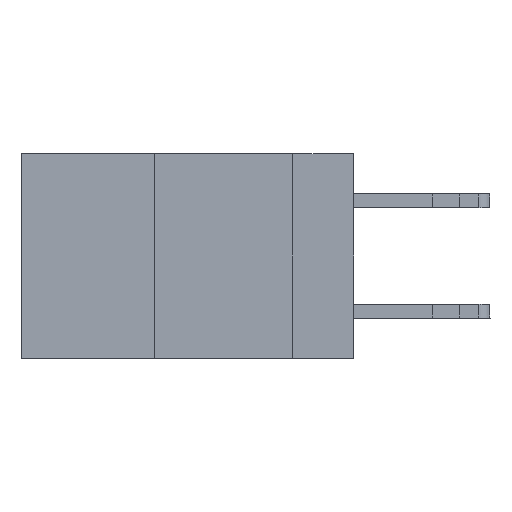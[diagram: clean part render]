
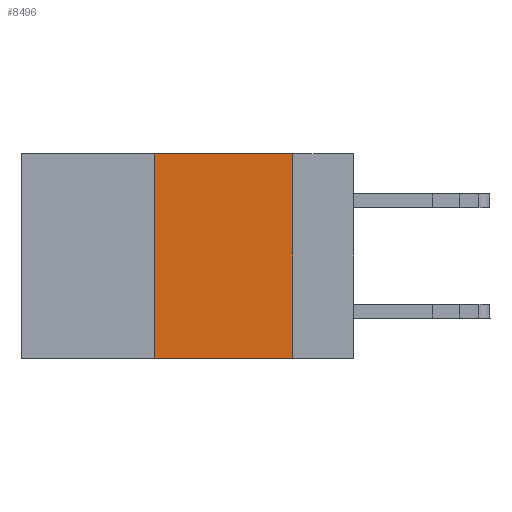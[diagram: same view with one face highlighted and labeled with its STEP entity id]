
A CAD part, left-side view. The second image highlights one B-rep face of the part: STEP entity #8496.
In plain terms, the highlighted planar face has unit normal (-1, 0, 0).
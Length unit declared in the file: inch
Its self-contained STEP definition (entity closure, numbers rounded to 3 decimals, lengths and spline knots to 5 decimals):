
#529 = CARTESIAN_POINT ( 'NONE',  ( 0., 0.36, 0. ) ) ;
#3308 = AXIS2_PLACEMENT_3D ( 'NONE', #15281, #18104, #31017 ) ;
#3557 = VERTEX_POINT ( 'NONE', #18134 ) ;
#4475 = CARTESIAN_POINT ( 'NONE',  ( 0., 0.6, 0. ) ) ;
#4531 = EDGE_LOOP ( 'NONE', ( #20678, #22236, #29000, #11725 ) ) ;
#5773 = VECTOR ( 'NONE', #17639, 39.37008 ) ;
#7805 = VECTOR ( 'NONE', #26830, 39.37008 ) ;
#8262 = LINE ( 'NONE', #529, #11926 ) ;
#8496 = ADVANCED_FACE ( 'NONE', ( #32356 ), #33274, .F. ) ;
#8916 = CARTESIAN_POINT ( 'NONE',  ( 0., 0.11, -0.37 ) ) ;
#10449 = DIRECTION ( 'NONE',  ( 0., 0., 1. ) ) ;
#11725 = ORIENTED_EDGE ( 'NONE', *, *, #25978, .T. ) ;
#11751 = EDGE_CURVE ( 'NONE', #28213, #17127, #28476, .T. ) ;
#11926 = VECTOR ( 'NONE', #10449, 39.37008 ) ;
#12063 = LINE ( 'NONE', #23306, #20612 ) ;
#15281 = CARTESIAN_POINT ( 'NONE',  ( 0., 0.6, 0. ) ) ;
#17127 = VERTEX_POINT ( 'NONE', #23658 ) ;
#17639 = DIRECTION ( 'NONE',  ( 0., -1., 0. ) ) ;
#18104 = DIRECTION ( 'NONE',  ( 1., 0., 0. ) ) ;
#18134 = CARTESIAN_POINT ( 'NONE',  ( 0., 0.36, -0.37 ) ) ;
#20462 = DIRECTION ( 'NONE',  ( 0., 0., -1. ) ) ;
#20612 = VECTOR ( 'NONE', #20462, 39.37008 ) ;
#20678 = ORIENTED_EDGE ( 'NONE', *, *, #23579, .F. ) ;
#22236 = ORIENTED_EDGE ( 'NONE', *, *, #11751, .F. ) ;
#23306 = CARTESIAN_POINT ( 'NONE',  ( 0., 0.11, 0. ) ) ;
#23579 = EDGE_CURVE ( 'NONE', #17127, #25927, #12063, .T. ) ;
#23658 = CARTESIAN_POINT ( 'NONE',  ( 0., 0.11, 0. ) ) ;
#25927 = VERTEX_POINT ( 'NONE', #8916 ) ;
#25978 = EDGE_CURVE ( 'NONE', #3557, #25927, #29318, .T. ) ;
#26830 = DIRECTION ( 'NONE',  ( 0., -1., 0. ) ) ;
#27222 = CARTESIAN_POINT ( 'NONE',  ( 0., 0.36, 0. ) ) ;
#28213 = VERTEX_POINT ( 'NONE', #27222 ) ;
#28476 = LINE ( 'NONE', #4475, #5773 ) ;
#29000 = ORIENTED_EDGE ( 'NONE', *, *, #29096, .F. ) ;
#29096 = EDGE_CURVE ( 'NONE', #3557, #28213, #8262, .T. ) ;
#29318 = LINE ( 'NONE', #31926, #7805 ) ;
#31017 = DIRECTION ( 'NONE',  ( 0., 0., -1. ) ) ;
#31926 = CARTESIAN_POINT ( 'NONE',  ( 0., 0.6, -0.37 ) ) ;
#32356 = FACE_OUTER_BOUND ( 'NONE', #4531, .T. ) ;
#33274 = PLANE ( 'NONE',  #3308 ) ;
